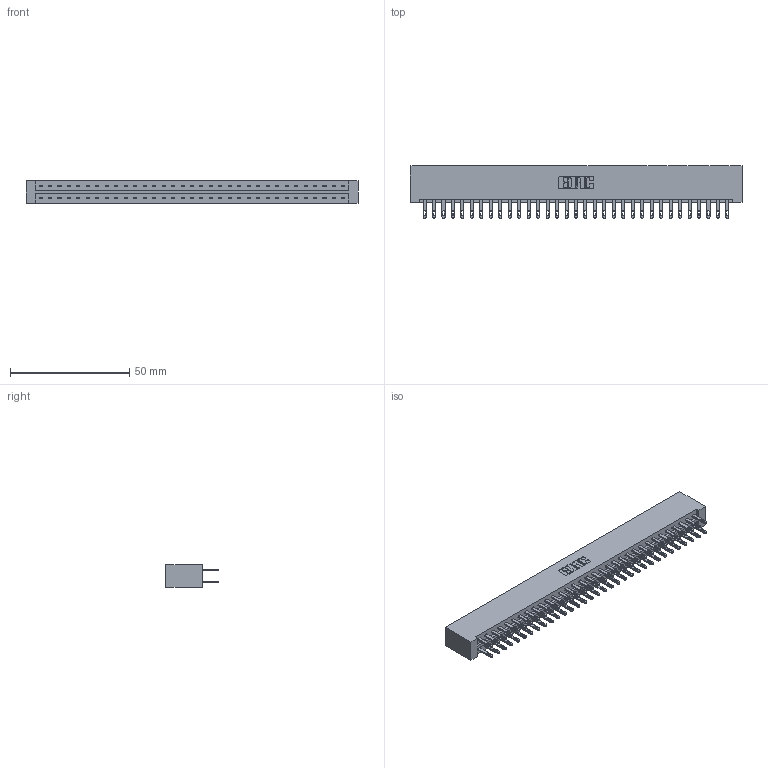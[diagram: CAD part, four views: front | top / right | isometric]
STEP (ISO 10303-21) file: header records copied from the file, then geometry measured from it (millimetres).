
FILE_DESCRIPTION (( 'STEP AP203' ), '1' );
FILE_NAME ('333-066-500-201.STEP', '2018-08-04T10:46:31', ( '' ), ( '' ), 'SwSTEP 2.0', 'SolidWorks 2016', '' );
FILE_SCHEMA (( 'CONFIG_CONTROL_DESIGN' ));
Length unit declared in the file: inch
Products named in the file (3): 333 Part_Lugless; 345-292-001_345-293-100; 333-066-500-201
Assembly tree (67 placements, depth 2):
  333-066-500-201
    333 Part_Lugless
    345-292-001_345-293-100  x66
Bounding box: 139.01 x 21.85 x 9.4 mm (x, y, z)
Volume: 14942.3 mm3; surface area: 18319.5 mm2
Topology: 67 solids, 67 shells, 3274 faces, 9989 edges, 6658 vertices
Faces by surface type: plane 2046, cylinder 1228
Entity records: 22047 total; most frequent: CARTESIAN_POINT 3662, ORIENTED_EDGE 3598, DIRECTION 3139, EDGE_CURVE 1799, VECTOR 1675, LINE 1675, VERTEX_POINT 1198, AXIS2_PLACEMENT_3D 732
